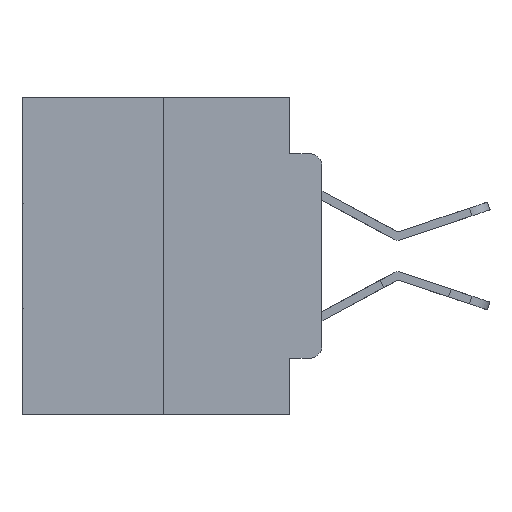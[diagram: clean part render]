
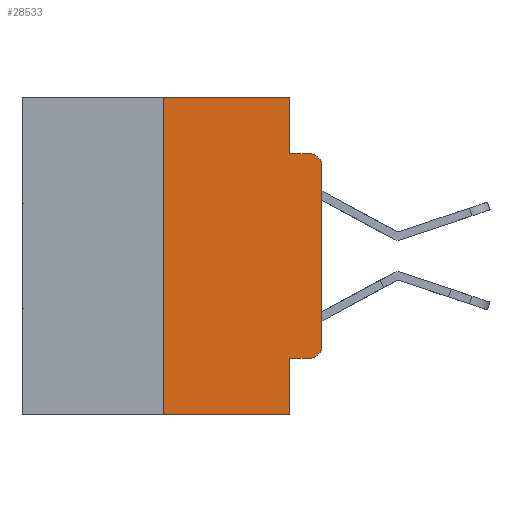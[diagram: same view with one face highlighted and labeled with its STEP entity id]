
A CAD part, left-side view. The second image highlights one B-rep face of the part: STEP entity #28533.
In plain terms, the highlighted planar face has unit normal (-1, 0, 0).
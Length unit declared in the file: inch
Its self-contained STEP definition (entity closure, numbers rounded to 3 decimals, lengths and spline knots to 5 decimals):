
#71 = CARTESIAN_POINT ( 'NONE',  ( 0., 0.02, -0.1085 ) ) ;
#75 = CARTESIAN_POINT ( 'NONE',  ( 0., 0.051, -0.4115 ) ) ;
#206 = DIRECTION ( 'NONE',  ( -1., 0., 0. ) ) ;
#701 = AXIS2_PLACEMENT_3D ( 'NONE', #71, #206, #20937 ) ;
#835 = CARTESIAN_POINT ( 'NONE',  ( 0., 0.02, -0.3915 ) ) ;
#1674 = LINE ( 'NONE', #21523, #25722 ) ;
#3085 = DIRECTION ( 'NONE',  ( 0., 0., -1. ) ) ;
#3317 = FACE_OUTER_BOUND ( 'NONE', #14629, .T. ) ;
#4441 = VECTOR ( 'NONE', #8226, 39.37008 ) ;
#4630 = CARTESIAN_POINT ( 'NONE',  ( 0., 0.051, 0. ) ) ;
#4917 = ORIENTED_EDGE ( 'NONE', *, *, #23761, .F. ) ;
#4934 = EDGE_CURVE ( 'NONE', #19561, #19205, #6950, .T. ) ;
#4949 = ORIENTED_EDGE ( 'NONE', *, *, #4934, .F. ) ;
#5182 = VECTOR ( 'NONE', #20918, 39.37008 ) ;
#5379 = CARTESIAN_POINT ( 'NONE',  ( 0., 0., -0.3915 ) ) ;
#5522 = DIRECTION ( 'NONE',  ( 0., -1., 0. ) ) ;
#5581 = DIRECTION ( 'NONE',  ( 0., -1., 0. ) ) ;
#5897 = EDGE_CURVE ( 'NONE', #25936, #16460, #7427, .T. ) ;
#6075 = CARTESIAN_POINT ( 'NONE',  ( 0., 0.25, 0. ) ) ;
#6232 = LINE ( 'NONE', #6603, #28102 ) ;
#6570 = VERTEX_POINT ( 'NONE', #5379 ) ;
#6603 = CARTESIAN_POINT ( 'NONE',  ( 0., 0.051, -0.0885 ) ) ;
#6622 = AXIS2_PLACEMENT_3D ( 'NONE', #835, #16632, #3085 ) ;
#6627 = VECTOR ( 'NONE', #5522, 39.37008 ) ;
#6918 = CARTESIAN_POINT ( 'NONE',  ( 0., 0.051, -0.5 ) ) ;
#6950 = LINE ( 'NONE', #10251, #22974 ) ;
#7176 = VERTEX_POINT ( 'NONE', #15544 ) ;
#7427 = CIRCLE ( 'NONE', #701, 0.02 ) ;
#8070 = DIRECTION ( 'NONE',  ( 1., 0., 0. ) ) ;
#8091 = ORIENTED_EDGE ( 'NONE', *, *, #26705, .F. ) ;
#8117 = EDGE_CURVE ( 'NONE', #19205, #16460, #6232, .T. ) ;
#8226 = DIRECTION ( 'NONE',  ( 0., 0., 1. ) ) ;
#9943 = CARTESIAN_POINT ( 'NONE',  ( 0., 0.02, -0.0885 ) ) ;
#10251 = CARTESIAN_POINT ( 'NONE',  ( 0., 0.051, 0. ) ) ;
#10357 = AXIS2_PLACEMENT_3D ( 'NONE', #21723, #8070, #23950 ) ;
#11832 = ORIENTED_EDGE ( 'NONE', *, *, #26658, .T. ) ;
#12673 = LINE ( 'NONE', #16716, #6627 ) ;
#12685 = CARTESIAN_POINT ( 'NONE',  ( 0., 0., 0. ) ) ;
#12912 = ORIENTED_EDGE ( 'NONE', *, *, #8117, .F. ) ;
#14629 = EDGE_LOOP ( 'NONE', ( #14940, #26504, #12912, #4949, #21820, #4917, #11832, #8091, #24285, #14965 ) ) ;
#14824 = PLANE ( 'NONE',  #10357 ) ;
#14906 = CARTESIAN_POINT ( 'NONE',  ( 0., 0.051, 0. ) ) ;
#14940 = ORIENTED_EDGE ( 'NONE', *, *, #27355, .T. ) ;
#14965 = ORIENTED_EDGE ( 'NONE', *, *, #22840, .T. ) ;
#15544 = CARTESIAN_POINT ( 'NONE',  ( 0., 0.25, -0.5 ) ) ;
#15996 = VERTEX_POINT ( 'NONE', #24253 ) ;
#16306 = CARTESIAN_POINT ( 'NONE',  ( 0., 0.051, -0.4115 ) ) ;
#16460 = VERTEX_POINT ( 'NONE', #9943 ) ;
#16632 = DIRECTION ( 'NONE',  ( -1., 0., 0. ) ) ;
#16716 = CARTESIAN_POINT ( 'NONE',  ( 0., 0.473, 0. ) ) ;
#16873 = LINE ( 'NONE', #14906, #24333 ) ;
#17174 = CARTESIAN_POINT ( 'NONE',  ( 0., 0.051, -0.0885 ) ) ;
#18098 = VERTEX_POINT ( 'NONE', #75 ) ;
#18140 = VERTEX_POINT ( 'NONE', #6918 ) ;
#18522 = DIRECTION ( 'NONE',  ( 0., 0., -1. ) ) ;
#19205 = VERTEX_POINT ( 'NONE', #17174 ) ;
#19561 = VERTEX_POINT ( 'NONE', #4630 ) ;
#19706 = DIRECTION ( 'NONE',  ( 0., 0., 1. ) ) ;
#20918 = DIRECTION ( 'NONE',  ( 0., -1., 0. ) ) ;
#20937 = DIRECTION ( 'NONE',  ( 0., 0., -1. ) ) ;
#21523 = CARTESIAN_POINT ( 'NONE',  ( 0., 0.473, -0.5 ) ) ;
#21723 = CARTESIAN_POINT ( 'NONE',  ( 0., 0.473, 0. ) ) ;
#21820 = ORIENTED_EDGE ( 'NONE', *, *, #25962, .F. ) ;
#21951 = CARTESIAN_POINT ( 'NONE',  ( 0., 0.25, 0. ) ) ;
#22558 = LINE ( 'NONE', #12685, #4441 ) ;
#22840 = EDGE_CURVE ( 'NONE', #15996, #6570, #22869, .T. ) ;
#22869 = CIRCLE ( 'NONE', #6622, 0.02 ) ;
#22974 = VECTOR ( 'NONE', #18522, 39.37008 ) ;
#23498 = CARTESIAN_POINT ( 'NONE',  ( 0., 0., -0.1085 ) ) ;
#23761 = EDGE_CURVE ( 'NONE', #7176, #27376, #28630, .T. ) ;
#23950 = DIRECTION ( 'NONE',  ( 0., 0., -1. ) ) ;
#24004 = LINE ( 'NONE', #16306, #5182 ) ;
#24191 = VECTOR ( 'NONE', #19706, 39.37008 ) ;
#24253 = CARTESIAN_POINT ( 'NONE',  ( 0., 0.02, -0.4115 ) ) ;
#24285 = ORIENTED_EDGE ( 'NONE', *, *, #26481, .T. ) ;
#24333 = VECTOR ( 'NONE', #28328, 39.37008 ) ;
#24738 = DIRECTION ( 'NONE',  ( 0., -1., 0. ) ) ;
#25722 = VECTOR ( 'NONE', #5581, 39.37008 ) ;
#25936 = VERTEX_POINT ( 'NONE', #23498 ) ;
#25962 = EDGE_CURVE ( 'NONE', #27376, #19561, #12673, .T. ) ;
#26481 = EDGE_CURVE ( 'NONE', #18098, #15996, #24004, .T. ) ;
#26504 = ORIENTED_EDGE ( 'NONE', *, *, #5897, .T. ) ;
#26658 = EDGE_CURVE ( 'NONE', #7176, #18140, #1674, .T. ) ;
#26705 = EDGE_CURVE ( 'NONE', #18098, #18140, #16873, .T. ) ;
#27355 = EDGE_CURVE ( 'NONE', #6570, #25936, #22558, .T. ) ;
#27376 = VERTEX_POINT ( 'NONE', #21951 ) ;
#28102 = VECTOR ( 'NONE', #24738, 39.37008 ) ;
#28328 = DIRECTION ( 'NONE',  ( 0., 0., -1. ) ) ;
#28533 = ADVANCED_FACE ( 'NONE', ( #3317 ), #14824, .F. ) ;
#28630 = LINE ( 'NONE', #6075, #24191 ) ;
